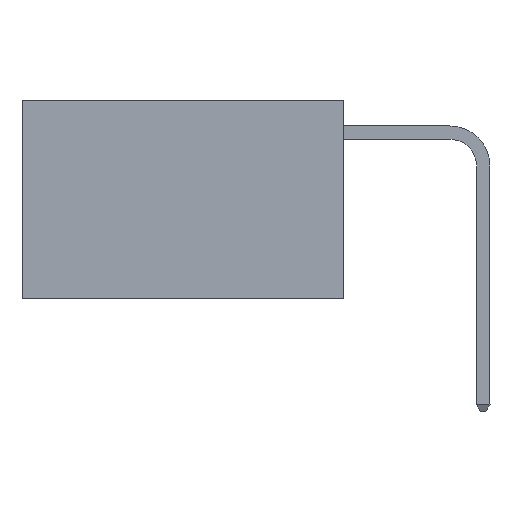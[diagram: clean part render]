
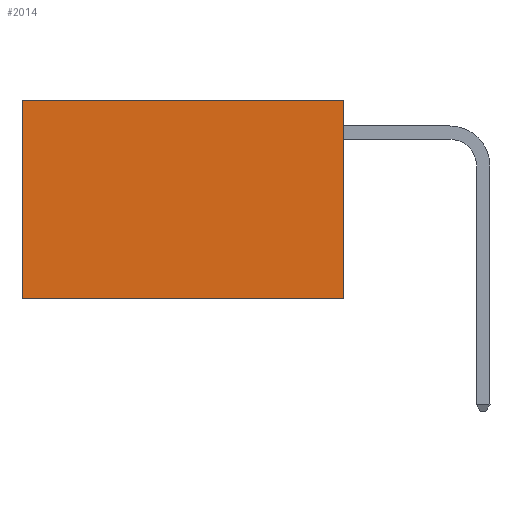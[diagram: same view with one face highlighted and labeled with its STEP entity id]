
A CAD part, left-side view. The second image highlights one B-rep face of the part: STEP entity #2014.
In plain terms, the highlighted planar face has unit normal (-1, 0, 0).
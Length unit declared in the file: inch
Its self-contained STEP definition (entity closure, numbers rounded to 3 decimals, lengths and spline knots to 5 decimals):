
#170 = VECTOR ( 'NONE', #3278, 39.37008 ) ;
#270 = VERTEX_POINT ( 'NONE', #1006 ) ;
#293 = DIRECTION ( 'NONE',  ( 1., 0., 0. ) ) ;
#427 = EDGE_CURVE ( 'NONE', #4599, #2737, #4764, .T. ) ;
#532 = DIRECTION ( 'NONE',  ( 0., 1., 0. ) ) ;
#914 = ORIENTED_EDGE ( 'NONE', *, *, #427, .F. ) ;
#1006 = CARTESIAN_POINT ( 'NONE',  ( 0.2625, 0.6, 0. ) ) ;
#1163 = CARTESIAN_POINT ( 'NONE',  ( 0.2625, 0., -0.37 ) ) ;
#1274 = ORIENTED_EDGE ( 'NONE', *, *, #6286, .T. ) ;
#1530 = LINE ( 'NONE', #2617, #6182 ) ;
#1828 = DIRECTION ( 'NONE',  ( 0., 1., 0. ) ) ;
#1948 = DIRECTION ( 'NONE',  ( 0., 0., -1. ) ) ;
#2014 = ADVANCED_FACE ( 'NONE', ( #3889 ), #5740, .F. ) ;
#2210 = EDGE_CURVE ( 'NONE', #5656, #4599, #1530, .T. ) ;
#2242 = EDGE_CURVE ( 'NONE', #270, #2737, #2571, .T. ) ;
#2571 = LINE ( 'NONE', #6843, #170 ) ;
#2617 = CARTESIAN_POINT ( 'NONE',  ( 0.2625, 0., 0. ) ) ;
#2737 = VERTEX_POINT ( 'NONE', #4342 ) ;
#2889 = VECTOR ( 'NONE', #1828, 39.37008 ) ;
#3278 = DIRECTION ( 'NONE',  ( 0., 0., -1. ) ) ;
#3889 = FACE_OUTER_BOUND ( 'NONE', #5047, .T. ) ;
#4342 = CARTESIAN_POINT ( 'NONE',  ( 0.2625, 0.6, -0.37 ) ) ;
#4599 = VERTEX_POINT ( 'NONE', #4676 ) ;
#4676 = CARTESIAN_POINT ( 'NONE',  ( 0.2625, 0., -0.37 ) ) ;
#4764 = LINE ( 'NONE', #1163, #5513 ) ;
#5047 = EDGE_LOOP ( 'NONE', ( #7688, #914, #5825, #1274 ) ) ;
#5185 = DIRECTION ( 'NONE',  ( 0., 0., -1. ) ) ;
#5513 = VECTOR ( 'NONE', #532, 39.37008 ) ;
#5656 = VERTEX_POINT ( 'NONE', #6655 ) ;
#5740 = PLANE ( 'NONE',  #7816 ) ;
#5825 = ORIENTED_EDGE ( 'NONE', *, *, #2210, .F. ) ;
#6182 = VECTOR ( 'NONE', #1948, 39.37008 ) ;
#6286 = EDGE_CURVE ( 'NONE', #5656, #270, #7246, .T. ) ;
#6655 = CARTESIAN_POINT ( 'NONE',  ( 0.2625, 0., 0. ) ) ;
#6664 = CARTESIAN_POINT ( 'NONE',  ( 0.2625, 0., 0. ) ) ;
#6843 = CARTESIAN_POINT ( 'NONE',  ( 0.2625, 0.6, 0. ) ) ;
#7246 = LINE ( 'NONE', #6664, #2889 ) ;
#7552 = CARTESIAN_POINT ( 'NONE',  ( 0.2625, 0., 0. ) ) ;
#7688 = ORIENTED_EDGE ( 'NONE', *, *, #2242, .T. ) ;
#7816 = AXIS2_PLACEMENT_3D ( 'NONE', #7552, #293, #5185 ) ;
